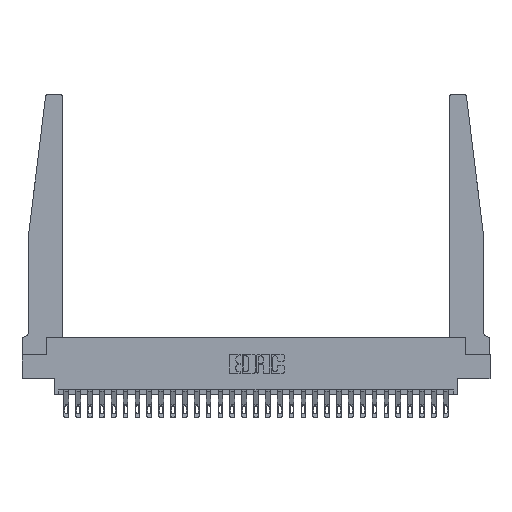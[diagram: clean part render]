
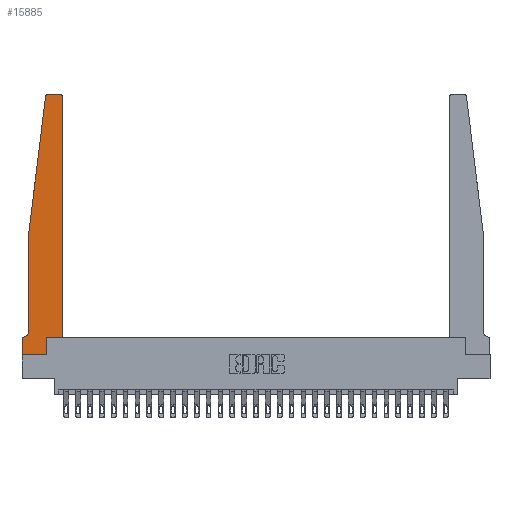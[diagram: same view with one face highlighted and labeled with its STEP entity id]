
A CAD part, top view. The second image highlights one B-rep face of the part: STEP entity #15885.
In plain terms, the highlighted planar face has unit normal (0, 0, 1).
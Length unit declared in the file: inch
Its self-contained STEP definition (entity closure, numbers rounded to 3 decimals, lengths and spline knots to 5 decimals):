
#43 = CARTESIAN_POINT ( 'NONE',  ( 0.015, 0.2375, 0.37 ) ) ;
#89 = AXIS2_PLACEMENT_3D ( 'NONE', #26331, #6966, #22123 ) ;
#244 = ORIENTED_EDGE ( 'NONE', *, *, #13901, .T. ) ;
#328 = ORIENTED_EDGE ( 'NONE', *, *, #8424, .T. ) ;
#353 = ORIENTED_EDGE ( 'NONE', *, *, #26434, .T. ) ;
#734 = CARTESIAN_POINT ( 'NONE',  ( 0., 0.1875, 0.37 ) ) ;
#773 = FACE_OUTER_BOUND ( 'NONE', #18495, .T. ) ;
#874 = VECTOR ( 'NONE', #17435, 39.37008 ) ;
#1468 = VECTOR ( 'NONE', #16520, 39.37008 ) ;
#1821 = DIRECTION ( 'NONE',  ( -0.122, -0.992, 0. ) ) ;
#1957 = CIRCLE ( 'NONE', #12932, 0.03 ) ;
#2070 = DIRECTION ( 'NONE',  ( 1., 0., 0. ) ) ;
#2172 = CARTESIAN_POINT ( 'NONE',  ( 0.065, 0.2375, 0.37 ) ) ;
#2177 = DIRECTION ( 'NONE',  ( -1., 0., 0. ) ) ;
#2184 = CARTESIAN_POINT ( 'NONE',  ( 0.24675, 2.72367, 0.37 ) ) ;
#2256 = CARTESIAN_POINT ( 'NONE',  ( 0.2605, 0.18, 0.37 ) ) ;
#2386 = VECTOR ( 'NONE', #3246, 39.37008 ) ;
#3025 = EDGE_CURVE ( 'NONE', #22889, #19711, #24434, .T. ) ;
#3246 = DIRECTION ( 'NONE',  ( 1., 0., 0. ) ) ;
#3503 = ORIENTED_EDGE ( 'NONE', *, *, #25753, .T. ) ;
#4113 = ORIENTED_EDGE ( 'NONE', *, *, #26055, .T. ) ;
#4964 = DIRECTION ( 'NONE',  ( 0., 0., 1. ) ) ;
#5078 = CARTESIAN_POINT ( 'NONE',  ( 0.395, 2.75, 0.37 ) ) ;
#6125 = VERTEX_POINT ( 'NONE', #12957 ) ;
#6242 = CARTESIAN_POINT ( 'NONE',  ( 0.065, 1.25, 0.37 ) ) ;
#6966 = DIRECTION ( 'NONE',  ( 0., 0., 1. ) ) ;
#7099 = EDGE_CURVE ( 'NONE', #15261, #17468, #27215, .T. ) ;
#7242 = LINE ( 'NONE', #25085, #1468 ) ;
#8155 = LINE ( 'NONE', #11893, #2386 ) ;
#8424 = EDGE_CURVE ( 'NONE', #18319, #11379, #7242, .T. ) ;
#8713 = VERTEX_POINT ( 'NONE', #15382 ) ;
#9035 = ORIENTED_EDGE ( 'NONE', *, *, #11857, .T. ) ;
#9398 = VERTEX_POINT ( 'NONE', #2184 ) ;
#9446 = VECTOR ( 'NONE', #27023, 39.37008 ) ;
#10078 = LINE ( 'NONE', #12703, #21627 ) ;
#10481 = CARTESIAN_POINT ( 'NONE',  ( 0.27653, 2.75, 0.37 ) ) ;
#10588 = DIRECTION ( 'NONE',  ( 0., -1., 0. ) ) ;
#10607 = CARTESIAN_POINT ( 'NONE',  ( 0.425, 0.18, 0.37 ) ) ;
#10963 = CARTESIAN_POINT ( 'NONE',  ( 0., 0., 0.37 ) ) ;
#10995 = ORIENTED_EDGE ( 'NONE', *, *, #25784, .T. ) ;
#11262 = AXIS2_PLACEMENT_3D ( 'NONE', #43, #15177, #2177 ) ;
#11379 = VERTEX_POINT ( 'NONE', #20104 ) ;
#11457 = VECTOR ( 'NONE', #14874, 39.37008 ) ;
#11857 = EDGE_CURVE ( 'NONE', #12259, #22889, #26326, .T. ) ;
#11893 = CARTESIAN_POINT ( 'NONE',  ( 0., 0., 0.37 ) ) ;
#11917 = CARTESIAN_POINT ( 'NONE',  ( 0.065, 0.1875, 0.37 ) ) ;
#12076 = EDGE_CURVE ( 'NONE', #17468, #9398, #25973, .T. ) ;
#12225 = CARTESIAN_POINT ( 'NONE',  ( 0.25, 2.75, 0.37 ) ) ;
#12259 = VERTEX_POINT ( 'NONE', #17923 ) ;
#12415 = ORIENTED_EDGE ( 'NONE', *, *, #20102, .T. ) ;
#12703 = CARTESIAN_POINT ( 'NONE',  ( 0., 0., 0.37 ) ) ;
#12932 = AXIS2_PLACEMENT_3D ( 'NONE', #17979, #4964, #20159 ) ;
#12957 = CARTESIAN_POINT ( 'NONE',  ( 0.2605, 0., 0.37 ) ) ;
#13212 = ORIENTED_EDGE ( 'NONE', *, *, #7099, .T. ) ;
#13901 = EDGE_CURVE ( 'NONE', #6125, #18319, #18173, .T. ) ;
#14006 = VECTOR ( 'NONE', #1821, 39.37008 ) ;
#14689 = LINE ( 'NONE', #27745, #14006 ) ;
#14835 = VECTOR ( 'NONE', #10588, 39.37008 ) ;
#14874 = DIRECTION ( 'NONE',  ( 0., 1., 0. ) ) ;
#15054 = DIRECTION ( 'NONE',  ( 0., 0., 1. ) ) ;
#15177 = DIRECTION ( 'NONE',  ( 0., 0., -1. ) ) ;
#15261 = VERTEX_POINT ( 'NONE', #5078 ) ;
#15382 = CARTESIAN_POINT ( 'NONE',  ( 0.425, 2.72, 0.37 ) ) ;
#15602 = PLANE ( 'NONE',  #89 ) ;
#15885 = ADVANCED_FACE ( 'NONE', ( #773 ), #15602, .T. ) ;
#16520 = DIRECTION ( 'NONE',  ( 1., 0., 0. ) ) ;
#17435 = DIRECTION ( 'NONE',  ( 0., 1., 0. ) ) ;
#17468 = VERTEX_POINT ( 'NONE', #10481 ) ;
#17562 = AXIS2_PLACEMENT_3D ( 'NONE', #27982, #15054, #2070 ) ;
#17923 = CARTESIAN_POINT ( 'NONE',  ( 0.065, 1.25, 0.37 ) ) ;
#17979 = CARTESIAN_POINT ( 'NONE',  ( 0.395, 2.72, 0.37 ) ) ;
#18173 = LINE ( 'NONE', #2256, #874 ) ;
#18319 = VERTEX_POINT ( 'NONE', #24093 ) ;
#18495 = EDGE_LOOP ( 'NONE', ( #13212, #25545, #12415, #9035, #27699, #4113, #3503, #19644, #244, #328, #10995, #353 ) ) ;
#19616 = VERTEX_POINT ( 'NONE', #10963 ) ;
#19644 = ORIENTED_EDGE ( 'NONE', *, *, #21929, .T. ) ;
#19711 = VERTEX_POINT ( 'NONE', #24201 ) ;
#20102 = EDGE_CURVE ( 'NONE', #9398, #12259, #14689, .T. ) ;
#20104 = CARTESIAN_POINT ( 'NONE',  ( 0.425, 0.18, 0.37 ) ) ;
#20159 = DIRECTION ( 'NONE',  ( 1., 0., 0. ) ) ;
#20308 = LINE ( 'NONE', #11917, #9446 ) ;
#20940 = LINE ( 'NONE', #10607, #11457 ) ;
#21627 = VECTOR ( 'NONE', #27807, 39.37008 ) ;
#21929 = EDGE_CURVE ( 'NONE', #19616, #6125, #8155, .T. ) ;
#22123 = DIRECTION ( 'NONE',  ( 1., 0., 0. ) ) ;
#22889 = VERTEX_POINT ( 'NONE', #2172 ) ;
#23015 = DIRECTION ( 'NONE',  ( -1., 0., 0. ) ) ;
#24093 = CARTESIAN_POINT ( 'NONE',  ( 0.2605, 0.18, 0.37 ) ) ;
#24201 = CARTESIAN_POINT ( 'NONE',  ( 0.015, 0.1875, 0.37 ) ) ;
#24434 = CIRCLE ( 'NONE', #11262, 0.05 ) ;
#25085 = CARTESIAN_POINT ( 'NONE',  ( 0.425, 0.18, 0.37 ) ) ;
#25545 = ORIENTED_EDGE ( 'NONE', *, *, #12076, .T. ) ;
#25753 = EDGE_CURVE ( 'NONE', #27101, #19616, #10078, .T. ) ;
#25784 = EDGE_CURVE ( 'NONE', #11379, #8713, #20940, .T. ) ;
#25973 = CIRCLE ( 'NONE', #17562, 0.03 ) ;
#26055 = EDGE_CURVE ( 'NONE', #19711, #27101, #20308, .T. ) ;
#26326 = LINE ( 'NONE', #6242, #14835 ) ;
#26331 = CARTESIAN_POINT ( 'NONE',  ( 0., 0.1875, 0.37 ) ) ;
#26434 = EDGE_CURVE ( 'NONE', #8713, #15261, #1957, .T. ) ;
#26544 = VECTOR ( 'NONE', #23015, 39.37008 ) ;
#27023 = DIRECTION ( 'NONE',  ( -1., 0., 0. ) ) ;
#27101 = VERTEX_POINT ( 'NONE', #734 ) ;
#27215 = LINE ( 'NONE', #12225, #26544 ) ;
#27699 = ORIENTED_EDGE ( 'NONE', *, *, #3025, .T. ) ;
#27745 = CARTESIAN_POINT ( 'NONE',  ( 0.065, 1.25, 0.37 ) ) ;
#27807 = DIRECTION ( 'NONE',  ( 0., -1., 0. ) ) ;
#27982 = CARTESIAN_POINT ( 'NONE',  ( 0.27653, 2.72, 0.37 ) ) ;
